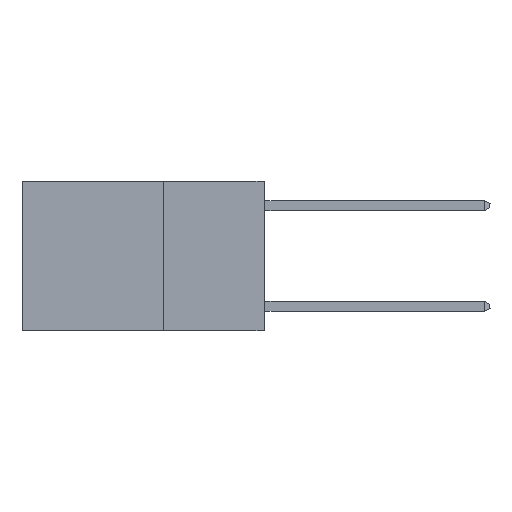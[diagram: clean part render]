
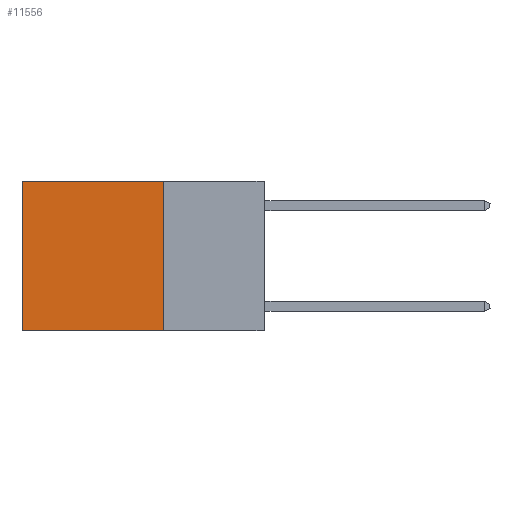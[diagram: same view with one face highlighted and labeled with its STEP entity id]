
A CAD part, left-side view. The second image highlights one B-rep face of the part: STEP entity #11556.
In plain terms, the highlighted planar face has unit normal (-1, 0, 0).
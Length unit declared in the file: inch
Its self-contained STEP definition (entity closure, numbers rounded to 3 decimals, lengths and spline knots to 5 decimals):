
#980 = FACE_OUTER_BOUND ( 'NONE', #19924, .T. ) ;
#1487 = VERTEX_POINT ( 'NONE', #13002 ) ;
#1855 = ORIENTED_EDGE ( 'NONE', *, *, #17614, .T. ) ;
#2391 = PLANE ( 'NONE',  #15063 ) ;
#2497 = CARTESIAN_POINT ( 'NONE',  ( 0.2625, 0.25, 0. ) ) ;
#2757 = DIRECTION ( 'NONE',  ( 0., 1., 0. ) ) ;
#2980 = VERTEX_POINT ( 'NONE', #18360 ) ;
#2997 = LINE ( 'NONE', #3097, #11944 ) ;
#3097 = CARTESIAN_POINT ( 'NONE',  ( 0.2625, 0.6, 0. ) ) ;
#4675 = LINE ( 'NONE', #10412, #7053 ) ;
#4975 = ORIENTED_EDGE ( 'NONE', *, *, #5787, .F. ) ;
#5451 = ORIENTED_EDGE ( 'NONE', *, *, #14913, .F. ) ;
#5765 = VERTEX_POINT ( 'NONE', #2497 ) ;
#5787 = EDGE_CURVE ( 'NONE', #5765, #7304, #19813, .T. ) ;
#5863 = DIRECTION ( 'NONE',  ( 1., 0., 0. ) ) ;
#7053 = VECTOR ( 'NONE', #13466, 39.37008 ) ;
#7304 = VERTEX_POINT ( 'NONE', #14223 ) ;
#8156 = ORIENTED_EDGE ( 'NONE', *, *, #12993, .T. ) ;
#10412 = CARTESIAN_POINT ( 'NONE',  ( 0.2625, 0.25, -0.37 ) ) ;
#10463 = DIRECTION ( 'NONE',  ( 0., 0., -1. ) ) ;
#11556 = ADVANCED_FACE ( 'NONE', ( #980 ), #2391, .F. ) ;
#11836 = VECTOR ( 'NONE', #10463, 39.37008 ) ;
#11944 = VECTOR ( 'NONE', #14213, 39.37008 ) ;
#12993 = EDGE_CURVE ( 'NONE', #2980, #1487, #2997, .T. ) ;
#13002 = CARTESIAN_POINT ( 'NONE',  ( 0.2625, 0.6, -0.37 ) ) ;
#13466 = DIRECTION ( 'NONE',  ( 0., 1., 0. ) ) ;
#13477 = CARTESIAN_POINT ( 'NONE',  ( 0.2625, 0.25, 0. ) ) ;
#13979 = VECTOR ( 'NONE', #2757, 39.37008 ) ;
#14213 = DIRECTION ( 'NONE',  ( 0., 0., -1. ) ) ;
#14223 = CARTESIAN_POINT ( 'NONE',  ( 0.2625, 0.25, -0.37 ) ) ;
#14733 = CARTESIAN_POINT ( 'NONE',  ( 0.2625, 0.25, 0. ) ) ;
#14913 = EDGE_CURVE ( 'NONE', #7304, #1487, #4675, .T. ) ;
#15063 = AXIS2_PLACEMENT_3D ( 'NONE', #14733, #5863, #18269 ) ;
#16860 = CARTESIAN_POINT ( 'NONE',  ( 0.2625, 0.25, 0. ) ) ;
#17614 = EDGE_CURVE ( 'NONE', #5765, #2980, #19565, .T. ) ;
#18269 = DIRECTION ( 'NONE',  ( 0., 0., -1. ) ) ;
#18360 = CARTESIAN_POINT ( 'NONE',  ( 0.2625, 0.6, 0. ) ) ;
#19565 = LINE ( 'NONE', #13477, #13979 ) ;
#19813 = LINE ( 'NONE', #16860, #11836 ) ;
#19924 = EDGE_LOOP ( 'NONE', ( #8156, #5451, #4975, #1855 ) ) ;
